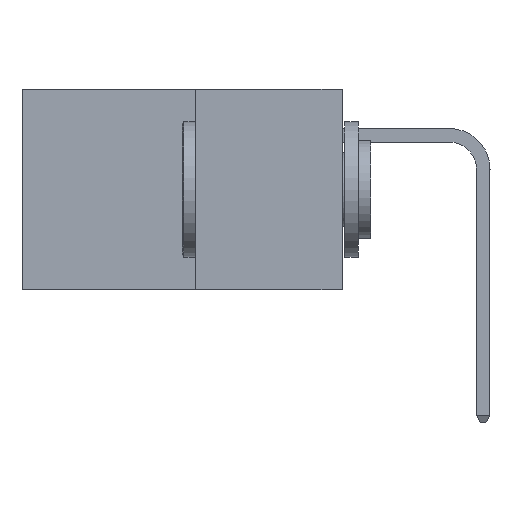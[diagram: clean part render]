
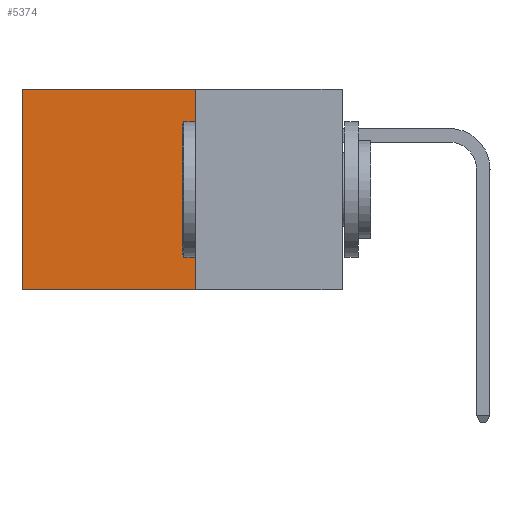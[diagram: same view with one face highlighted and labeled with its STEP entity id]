
A CAD part, left-side view. The second image highlights one B-rep face of the part: STEP entity #5374.
In plain terms, the highlighted planar face has unit normal (-1, 0, 0).
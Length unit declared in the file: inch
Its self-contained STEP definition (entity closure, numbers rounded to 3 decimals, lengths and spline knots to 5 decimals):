
#58 = VERTEX_POINT ( 'NONE', #1590 ) ;
#458 = ORIENTED_EDGE ( 'NONE', *, *, #6444, .T. ) ;
#953 = VECTOR ( 'NONE', #3379, 39.37008 ) ;
#1022 = DIRECTION ( 'NONE',  ( 0., 0., -1. ) ) ;
#1090 = EDGE_CURVE ( 'NONE', #5667, #1335, #4614, .T. ) ;
#1129 = CARTESIAN_POINT ( 'NONE',  ( 0.277, 0.27, -0.37 ) ) ;
#1335 = VERTEX_POINT ( 'NONE', #3497 ) ;
#1456 = CARTESIAN_POINT ( 'NONE',  ( 0.277, 0.27, -0.37 ) ) ;
#1590 = CARTESIAN_POINT ( 'NONE',  ( 0.277, 0.59, 0. ) ) ;
#1921 = AXIS2_PLACEMENT_3D ( 'NONE', #8846, #8696, #8644 ) ;
#1976 = VECTOR ( 'NONE', #2902, 39.37008 ) ;
#2120 = EDGE_LOOP ( 'NONE', ( #458, #7924, #2719, #6446 ) ) ;
#2150 = CARTESIAN_POINT ( 'NONE',  ( 0.277, 0.59, -0.37 ) ) ;
#2719 = ORIENTED_EDGE ( 'NONE', *, *, #6030, .F. ) ;
#2746 = VERTEX_POINT ( 'NONE', #6807 ) ;
#2829 = LINE ( 'NONE', #4301, #6550 ) ;
#2902 = DIRECTION ( 'NONE',  ( 0., 1., 0. ) ) ;
#3029 = FACE_OUTER_BOUND ( 'NONE', #2120, .T. ) ;
#3156 = LINE ( 'NONE', #2150, #6636 ) ;
#3379 = DIRECTION ( 'NONE',  ( 0., 1., 0. ) ) ;
#3497 = CARTESIAN_POINT ( 'NONE',  ( 0.277, 0.59, -0.37 ) ) ;
#3915 = LINE ( 'NONE', #7940, #1976 ) ;
#4291 = DIRECTION ( 'NONE',  ( 0., 0., -1. ) ) ;
#4301 = CARTESIAN_POINT ( 'NONE',  ( 0.277, 0.27, -0.37 ) ) ;
#4614 = LINE ( 'NONE', #1129, #953 ) ;
#5374 = ADVANCED_FACE ( 'NONE', ( #3029 ), #8892, .F. ) ;
#5667 = VERTEX_POINT ( 'NONE', #1456 ) ;
#5729 = EDGE_CURVE ( 'NONE', #2746, #58, #3915, .T. ) ;
#6030 = EDGE_CURVE ( 'NONE', #2746, #5667, #2829, .T. ) ;
#6444 = EDGE_CURVE ( 'NONE', #58, #1335, #3156, .T. ) ;
#6446 = ORIENTED_EDGE ( 'NONE', *, *, #5729, .T. ) ;
#6550 = VECTOR ( 'NONE', #4291, 39.37008 ) ;
#6636 = VECTOR ( 'NONE', #1022, 39.37008 ) ;
#6807 = CARTESIAN_POINT ( 'NONE',  ( 0.277, 0.27, 0. ) ) ;
#7924 = ORIENTED_EDGE ( 'NONE', *, *, #1090, .F. ) ;
#7940 = CARTESIAN_POINT ( 'NONE',  ( 0.277, 0.27, 0. ) ) ;
#8644 = DIRECTION ( 'NONE',  ( 0., 0., -1. ) ) ;
#8696 = DIRECTION ( 'NONE',  ( 1., 0., 0. ) ) ;
#8846 = CARTESIAN_POINT ( 'NONE',  ( 0.277, 0.27, -0.37 ) ) ;
#8892 = PLANE ( 'NONE',  #1921 ) ;
